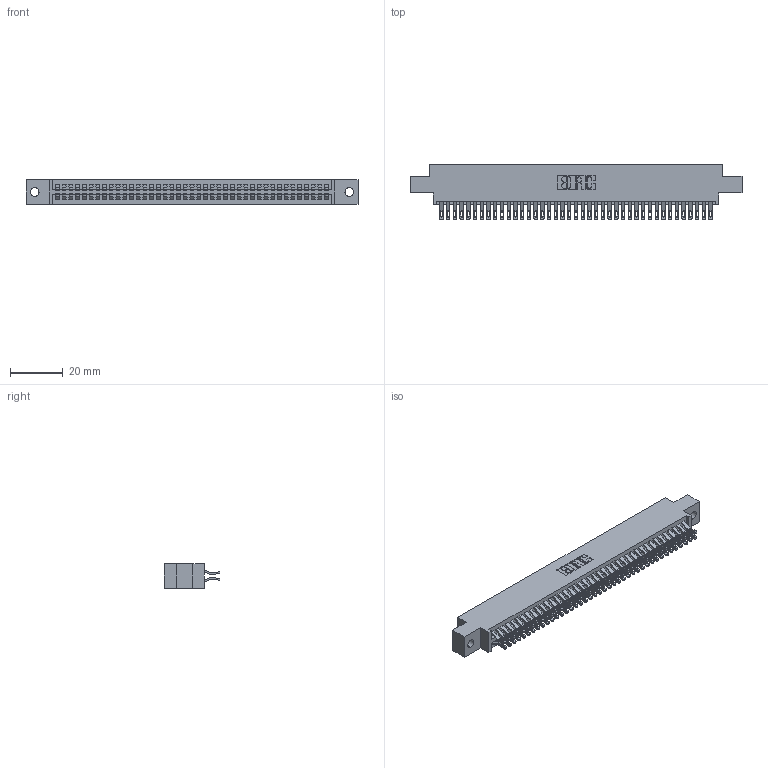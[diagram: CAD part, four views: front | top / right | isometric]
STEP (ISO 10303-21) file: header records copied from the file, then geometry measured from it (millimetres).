
FILE_DESCRIPTION (( 'STEP AP203' ), '1' );
FILE_NAME ('395-082-555-802.STEP', '2019-10-25T07:13:03', ( '' ), ( '' ), 'SwSTEP 2.0', 'SolidWorks 2016', '' );
FILE_SCHEMA (( 'CONFIG_CONTROL_DESIGN' ));
Length unit declared in the file: inch
Products named in the file (3): 345 Part_0.170 Offset - 0.128 Dia; 345-292-001_555 Tail; 395-082-555-802
Assembly tree (83 placements, depth 2):
  395-082-555-802
    345 Part_0.170 Offset - 0.128 Dia
    345-292-001_555 Tail  x82
Bounding box: 125.35 x 21.13 x 9.4 mm (x, y, z)
Volume: 12255 mm3; surface area: 18793.6 mm2
Topology: 83 solids, 83 shells, 4722 faces, 14867 edges, 9910 vertices
Faces by surface type: plane 2626, cylinder 2096
Entity records: 32765 total; most frequent: CARTESIAN_POINT 5530, ORIENTED_EDGE 5434, DIRECTION 4845, EDGE_CURVE 2717, LINE 2401, VECTOR 2401, VERTEX_POINT 1810, AXIS2_PLACEMENT_3D 1222
